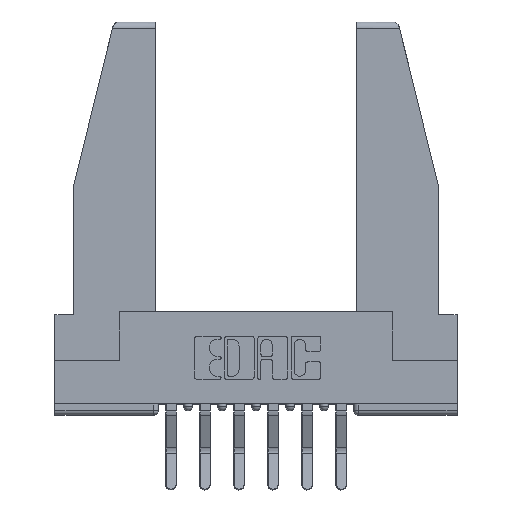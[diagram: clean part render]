
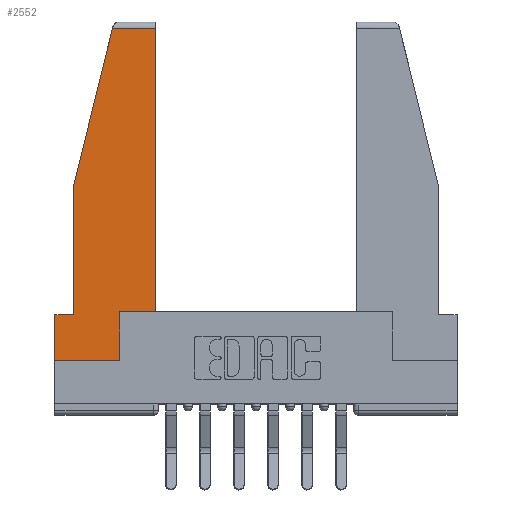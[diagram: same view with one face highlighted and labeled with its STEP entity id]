
A CAD part, top view. The second image highlights one B-rep face of the part: STEP entity #2552.
In plain terms, the highlighted planar face has unit normal (0, 0, 1).
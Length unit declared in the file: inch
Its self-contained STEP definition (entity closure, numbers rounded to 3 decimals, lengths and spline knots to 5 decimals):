
#38 = CARTESIAN_POINT ( 'NONE',  ( 0., 0.21, 0. ) ) ;
#403 = VECTOR ( 'NONE', #2926, 39.37008 ) ;
#479 = ORIENTED_EDGE ( 'NONE', *, *, #10672, .T. ) ;
#643 = VECTOR ( 'NONE', #4681, 39.37008 ) ;
#736 = VERTEX_POINT ( 'NONE', #2388 ) ;
#776 = CARTESIAN_POINT ( 'NONE',  ( 0., 0.21, 0. ) ) ;
#778 = PLANE ( 'NONE',  #3895 ) ;
#800 = VERTEX_POINT ( 'NONE', #2597 ) ;
#910 = VERTEX_POINT ( 'NONE', #8850 ) ;
#1421 = VERTEX_POINT ( 'NONE', #12202 ) ;
#1804 = EDGE_CURVE ( 'NONE', #5767, #800, #2172, .T. ) ;
#1838 = CARTESIAN_POINT ( 'NONE',  ( 0.461, 0.223, 0. ) ) ;
#1887 = ORIENTED_EDGE ( 'NONE', *, *, #8757, .T. ) ;
#2172 = LINE ( 'NONE', #2327, #8460 ) ;
#2327 = CARTESIAN_POINT ( 'NONE',  ( 0.086, 0.8, 0. ) ) ;
#2388 = CARTESIAN_POINT ( 'NONE',  ( 0.297, 0.223, 0. ) ) ;
#2552 = ADVANCED_FACE ( 'NONE', ( #5777 ), #778, .T. ) ;
#2597 = CARTESIAN_POINT ( 'NONE',  ( 0.086, 0.21, 0. ) ) ;
#2763 = EDGE_CURVE ( 'NONE', #910, #1421, #9169, .T. ) ;
#2926 = DIRECTION ( 'NONE',  ( -1., 0., 0. ) ) ;
#3371 = VECTOR ( 'NONE', #3869, 39.37008 ) ;
#3462 = EDGE_LOOP ( 'NONE', ( #479, #8949, #5694, #6270, #1887, #10835, #5819, #5161, #7474 ) ) ;
#3834 = CARTESIAN_POINT ( 'NONE',  ( 0., 0., 0. ) ) ;
#3869 = DIRECTION ( 'NONE',  ( 0., 1., 0. ) ) ;
#3895 = AXIS2_PLACEMENT_3D ( 'NONE', #3834, #5848, #7342 ) ;
#4380 = VERTEX_POINT ( 'NONE', #11147 ) ;
#4563 = LINE ( 'NONE', #4896, #11822 ) ;
#4681 = DIRECTION ( 'NONE',  ( -1., 0., 0. ) ) ;
#4777 = CARTESIAN_POINT ( 'NONE',  ( 0., 1.52, 0. ) ) ;
#4896 = CARTESIAN_POINT ( 'NONE',  ( 0.297, 0.223, 0. ) ) ;
#5161 = ORIENTED_EDGE ( 'NONE', *, *, #6463, .T. ) ;
#5373 = EDGE_CURVE ( 'NONE', #736, #4380, #4563, .T. ) ;
#5418 = DIRECTION ( 'NONE',  ( 0., 1., 0. ) ) ;
#5434 = DIRECTION ( 'NONE',  ( 0., -1., 0. ) ) ;
#5449 = CARTESIAN_POINT ( 'NONE',  ( 0.297, 0., 0. ) ) ;
#5520 = CARTESIAN_POINT ( 'NONE',  ( 0.461, 1.52, 0. ) ) ;
#5603 = VECTOR ( 'NONE', #5418, 39.37008 ) ;
#5655 = DIRECTION ( 'NONE',  ( 0., -1., 0. ) ) ;
#5694 = ORIENTED_EDGE ( 'NONE', *, *, #11064, .T. ) ;
#5767 = VERTEX_POINT ( 'NONE', #6373 ) ;
#5777 = FACE_OUTER_BOUND ( 'NONE', #3462, .T. ) ;
#5786 = EDGE_CURVE ( 'NONE', #1421, #10041, #11216, .T. ) ;
#5819 = ORIENTED_EDGE ( 'NONE', *, *, #5786, .T. ) ;
#5848 = DIRECTION ( 'NONE',  ( 0., 0., 1. ) ) ;
#5905 = LINE ( 'NONE', #8188, #11220 ) ;
#5921 = LINE ( 'NONE', #1838, #3371 ) ;
#6270 = ORIENTED_EDGE ( 'NONE', *, *, #1804, .T. ) ;
#6326 = DIRECTION ( 'NONE',  ( 1., 0., 0. ) ) ;
#6373 = CARTESIAN_POINT ( 'NONE',  ( 0.086, 0.8, 0. ) ) ;
#6463 = EDGE_CURVE ( 'NONE', #10041, #736, #12108, .T. ) ;
#6566 = EDGE_CURVE ( 'NONE', #8658, #8996, #7068, .T. ) ;
#7068 = LINE ( 'NONE', #4777, #643 ) ;
#7342 = DIRECTION ( 'NONE',  ( 1., 0., 0. ) ) ;
#7474 = ORIENTED_EDGE ( 'NONE', *, *, #5373, .T. ) ;
#8004 = DIRECTION ( 'NONE',  ( 1., 0., 0. ) ) ;
#8120 = VECTOR ( 'NONE', #6326, 39.37008 ) ;
#8188 = CARTESIAN_POINT ( 'NONE',  ( 0.271, 1.55, 0. ) ) ;
#8460 = VECTOR ( 'NONE', #5655, 39.37008 ) ;
#8658 = VERTEX_POINT ( 'NONE', #5520 ) ;
#8757 = EDGE_CURVE ( 'NONE', #800, #910, #11417, .T. ) ;
#8850 = CARTESIAN_POINT ( 'NONE',  ( 0., 0.21, 0. ) ) ;
#8949 = ORIENTED_EDGE ( 'NONE', *, *, #6566, .T. ) ;
#8996 = VERTEX_POINT ( 'NONE', #11637 ) ;
#9169 = LINE ( 'NONE', #776, #10760 ) ;
#10041 = VERTEX_POINT ( 'NONE', #11299 ) ;
#10672 = EDGE_CURVE ( 'NONE', #4380, #8658, #5921, .T. ) ;
#10760 = VECTOR ( 'NONE', #5434, 39.37008 ) ;
#10835 = ORIENTED_EDGE ( 'NONE', *, *, #2763, .T. ) ;
#11064 = EDGE_CURVE ( 'NONE', #8996, #5767, #5905, .T. ) ;
#11140 = DIRECTION ( 'NONE',  ( -0.239, -0.971, 0. ) ) ;
#11147 = CARTESIAN_POINT ( 'NONE',  ( 0.461, 0.223, 0. ) ) ;
#11216 = LINE ( 'NONE', #11998, #8120 ) ;
#11220 = VECTOR ( 'NONE', #11140, 39.37008 ) ;
#11299 = CARTESIAN_POINT ( 'NONE',  ( 0.297, 0., 0. ) ) ;
#11417 = LINE ( 'NONE', #38, #403 ) ;
#11637 = CARTESIAN_POINT ( 'NONE',  ( 0.2636, 1.52, 0. ) ) ;
#11822 = VECTOR ( 'NONE', #8004, 39.37008 ) ;
#11998 = CARTESIAN_POINT ( 'NONE',  ( 0., 0., 0. ) ) ;
#12108 = LINE ( 'NONE', #5449, #5603 ) ;
#12202 = CARTESIAN_POINT ( 'NONE',  ( 0., 0., 0. ) ) ;
